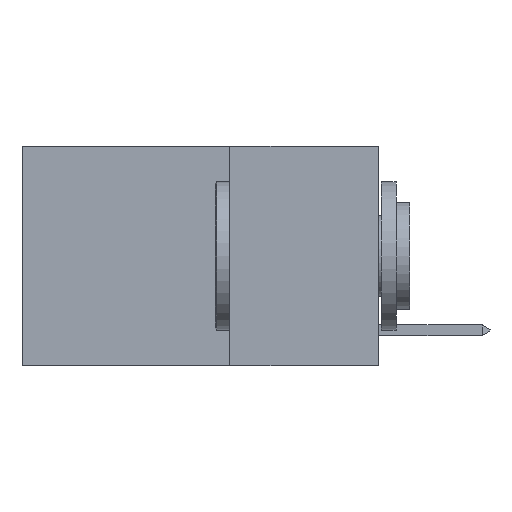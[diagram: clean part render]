
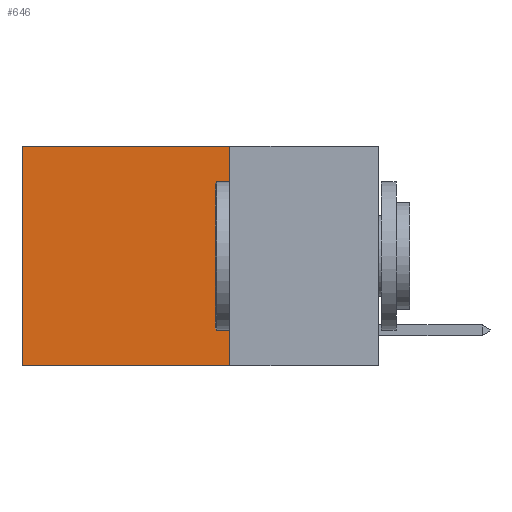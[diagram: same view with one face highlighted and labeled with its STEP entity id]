
A CAD part, left-side view. The second image highlights one B-rep face of the part: STEP entity #646.
In plain terms, the highlighted planar face has unit normal (-1, 0, 0).
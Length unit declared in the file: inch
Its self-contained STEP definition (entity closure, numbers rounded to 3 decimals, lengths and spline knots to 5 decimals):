
#249 = LINE ( 'NONE', #4018, #7206 ) ;
#646 = ADVANCED_FACE ( 'NONE', ( #6750 ), #6092, .F. ) ;
#790 = ORIENTED_EDGE ( 'NONE', *, *, #8763, .T. ) ;
#895 = EDGE_LOOP ( 'NONE', ( #4895, #3921, #9222, #790 ) ) ;
#1110 = VERTEX_POINT ( 'NONE', #5326 ) ;
#1158 = VERTEX_POINT ( 'NONE', #4682 ) ;
#1471 = CARTESIAN_POINT ( 'NONE',  ( 0.2625, 0.6, 0. ) ) ;
#1791 = CARTESIAN_POINT ( 'NONE',  ( 0.2625, 0.6, 0. ) ) ;
#1952 = VECTOR ( 'NONE', #5053, 39.37008 ) ;
#2382 = CARTESIAN_POINT ( 'NONE',  ( 0.2625, 0.25, 0. ) ) ;
#2434 = LINE ( 'NONE', #2382, #6162 ) ;
#2464 = CARTESIAN_POINT ( 'NONE',  ( 0.2625, 0.25, 0. ) ) ;
#2802 = CARTESIAN_POINT ( 'NONE',  ( 0.2625, 0.25, -0.37 ) ) ;
#3263 = EDGE_CURVE ( 'NONE', #8412, #1110, #2434, .T. ) ;
#3921 = ORIENTED_EDGE ( 'NONE', *, *, #5509, .F. ) ;
#4018 = CARTESIAN_POINT ( 'NONE',  ( 0.2625, 0.25, 0. ) ) ;
#4444 = LINE ( 'NONE', #1471, #1952 ) ;
#4682 = CARTESIAN_POINT ( 'NONE',  ( 0.2625, 0.6, -0.37 ) ) ;
#4895 = ORIENTED_EDGE ( 'NONE', *, *, #9041, .T. ) ;
#5053 = DIRECTION ( 'NONE',  ( 0., 0., -1. ) ) ;
#5075 = LINE ( 'NONE', #2802, #8637 ) ;
#5326 = CARTESIAN_POINT ( 'NONE',  ( 0.2625, 0.25, -0.37 ) ) ;
#5336 = DIRECTION ( 'NONE',  ( 0., 0., -1. ) ) ;
#5509 = EDGE_CURVE ( 'NONE', #1110, #1158, #5075, .T. ) ;
#6092 = PLANE ( 'NONE',  #9291 ) ;
#6141 = VERTEX_POINT ( 'NONE', #1791 ) ;
#6162 = VECTOR ( 'NONE', #7554, 39.37008 ) ;
#6338 = CARTESIAN_POINT ( 'NONE',  ( 0.2625, 0.25, 0. ) ) ;
#6750 = FACE_OUTER_BOUND ( 'NONE', #895, .T. ) ;
#7206 = VECTOR ( 'NONE', #8995, 39.37008 ) ;
#7554 = DIRECTION ( 'NONE',  ( 0., 0., -1. ) ) ;
#7973 = DIRECTION ( 'NONE',  ( 0., 1., 0. ) ) ;
#8412 = VERTEX_POINT ( 'NONE', #6338 ) ;
#8637 = VECTOR ( 'NONE', #7973, 39.37008 ) ;
#8763 = EDGE_CURVE ( 'NONE', #8412, #6141, #249, .T. ) ;
#8949 = DIRECTION ( 'NONE',  ( 1., 0., 0. ) ) ;
#8995 = DIRECTION ( 'NONE',  ( 0., 1., 0. ) ) ;
#9041 = EDGE_CURVE ( 'NONE', #6141, #1158, #4444, .T. ) ;
#9222 = ORIENTED_EDGE ( 'NONE', *, *, #3263, .F. ) ;
#9291 = AXIS2_PLACEMENT_3D ( 'NONE', #2464, #8949, #5336 ) ;
